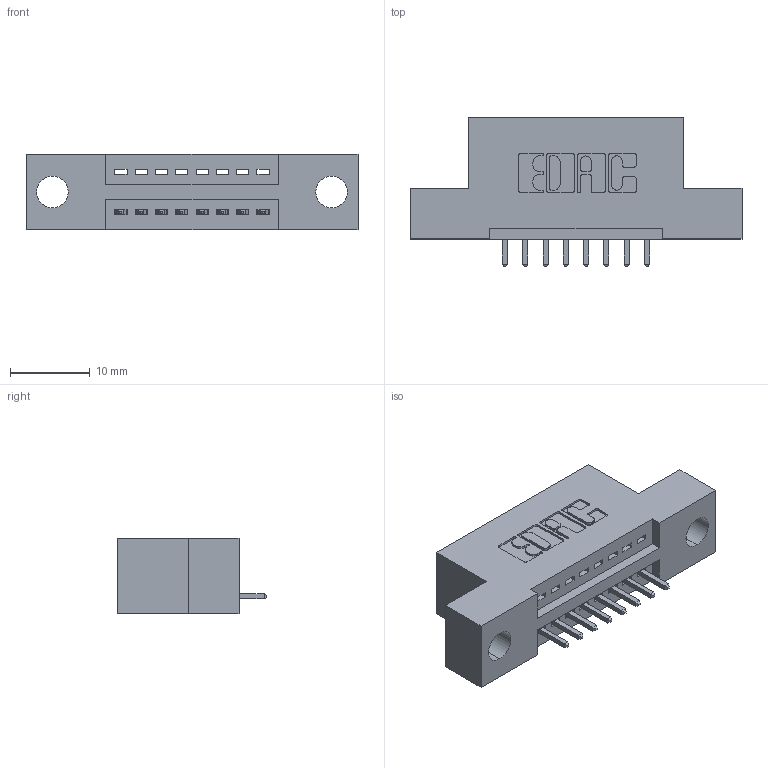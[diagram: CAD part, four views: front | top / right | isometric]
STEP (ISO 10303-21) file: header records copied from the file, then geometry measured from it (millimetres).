
FILE_DESCRIPTION (( 'STEP AP203' ), '1' );
FILE_NAME ('345-008-521-104.STEP', '2021-05-26T14:02:32', ( '' ), ( '' ), 'SwSTEP 2.0', 'SolidWorks 2020', '' );
FILE_SCHEMA (( 'CONFIG_CONTROL_DESIGN' ));
Length unit declared in the file: inch
Products named in the file (3): 345-008-521-104; 345-292-001_345-293-121; 345 Part_Flush Mounting Lugs - 0.156 Dia-TI
Assembly tree (9 placements, depth 2):
  345-008-521-104
    345 Part_Flush Mounting Lugs - 0.156 Dia-TI
    345-292-001_345-293-121  x8
Bounding box: 41.53 x 18.72 x 9.4 mm (x, y, z)
Volume: 3537.2 mm3; surface area: 3992 mm2
Topology: 9 solids, 9 shells, 604 faces, 1785 edges, 1178 vertices
Faces by surface type: plane 414, cylinder 190
Entity records: 11035 total; most frequent: CARTESIAN_POINT 1922, ORIENTED_EDGE 1862, DIRECTION 1727, EDGE_CURVE 931, VECTOR 767, LINE 767, VERTEX_POINT 618, AXIS2_PLACEMENT_3D 480
